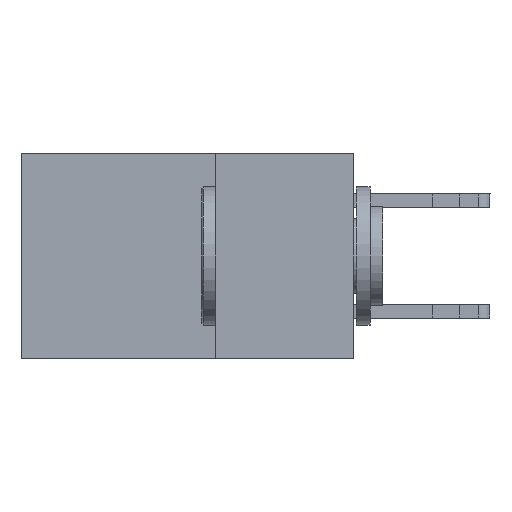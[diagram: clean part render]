
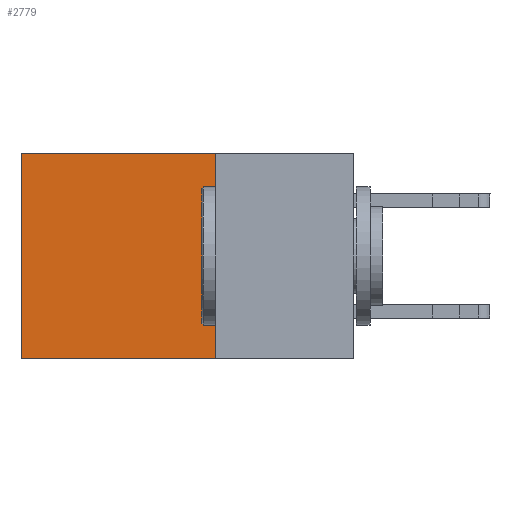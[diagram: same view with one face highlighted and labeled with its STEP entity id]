
A CAD part, left-side view. The second image highlights one B-rep face of the part: STEP entity #2779.
In plain terms, the highlighted planar face has unit normal (-1, 0, 0).
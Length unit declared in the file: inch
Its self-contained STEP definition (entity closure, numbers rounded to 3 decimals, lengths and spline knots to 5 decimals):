
#341 = EDGE_CURVE ( 'NONE', #2860, #11975, #12820, .T. ) ;
#876 = ORIENTED_EDGE ( 'NONE', *, *, #341, .T. ) ;
#2378 = VECTOR ( 'NONE', #12838, 39.37008 ) ;
#2779 = ADVANCED_FACE ( 'NONE', ( #11607 ), #12449, .F. ) ;
#2860 = VERTEX_POINT ( 'NONE', #17857 ) ;
#3425 = ORIENTED_EDGE ( 'NONE', *, *, #19374, .F. ) ;
#4796 = CARTESIAN_POINT ( 'NONE',  ( 0.2875, 0.25, -0.37 ) ) ;
#5244 = EDGE_CURVE ( 'NONE', #7590, #14618, #22636, .T. ) ;
#6620 = VECTOR ( 'NONE', #10534, 39.37008 ) ;
#6701 = CARTESIAN_POINT ( 'NONE',  ( 0.2875, 0.25, 0. ) ) ;
#6959 = CARTESIAN_POINT ( 'NONE',  ( 0.2875, 0.6, 0. ) ) ;
#7257 = CARTESIAN_POINT ( 'NONE',  ( 0.2875, 0.6, 0. ) ) ;
#7590 = VERTEX_POINT ( 'NONE', #20749 ) ;
#7975 = VECTOR ( 'NONE', #23348, 39.37008 ) ;
#9350 = EDGE_LOOP ( 'NONE', ( #12861, #20910, #3425, #876 ) ) ;
#9606 = CARTESIAN_POINT ( 'NONE',  ( 0.2875, 0.6, -0.37 ) ) ;
#9964 = CARTESIAN_POINT ( 'NONE',  ( 0.2875, 0.25, 0. ) ) ;
#9969 = LINE ( 'NONE', #7257, #2378 ) ;
#10534 = DIRECTION ( 'NONE',  ( 0., 1., 0. ) ) ;
#11607 = FACE_OUTER_BOUND ( 'NONE', #9350, .T. ) ;
#11975 = VERTEX_POINT ( 'NONE', #6959 ) ;
#12315 = EDGE_CURVE ( 'NONE', #11975, #14618, #9969, .T. ) ;
#12449 = PLANE ( 'NONE',  #23712 ) ;
#12719 = DIRECTION ( 'NONE',  ( 1., 0., 0. ) ) ;
#12820 = LINE ( 'NONE', #18076, #15816 ) ;
#12838 = DIRECTION ( 'NONE',  ( 0., 0., -1. ) ) ;
#12861 = ORIENTED_EDGE ( 'NONE', *, *, #12315, .T. ) ;
#14494 = DIRECTION ( 'NONE',  ( 0., 0., -1. ) ) ;
#14618 = VERTEX_POINT ( 'NONE', #9606 ) ;
#15816 = VECTOR ( 'NONE', #16187, 39.37008 ) ;
#16187 = DIRECTION ( 'NONE',  ( 0., 1., 0. ) ) ;
#17077 = LINE ( 'NONE', #9964, #7975 ) ;
#17857 = CARTESIAN_POINT ( 'NONE',  ( 0.2875, 0.25, 0. ) ) ;
#18076 = CARTESIAN_POINT ( 'NONE',  ( 0.2875, 0.25, 0. ) ) ;
#19374 = EDGE_CURVE ( 'NONE', #2860, #7590, #17077, .T. ) ;
#20749 = CARTESIAN_POINT ( 'NONE',  ( 0.2875, 0.25, -0.37 ) ) ;
#20910 = ORIENTED_EDGE ( 'NONE', *, *, #5244, .F. ) ;
#22636 = LINE ( 'NONE', #4796, #6620 ) ;
#23348 = DIRECTION ( 'NONE',  ( 0., 0., -1. ) ) ;
#23712 = AXIS2_PLACEMENT_3D ( 'NONE', #6701, #12719, #14494 ) ;
